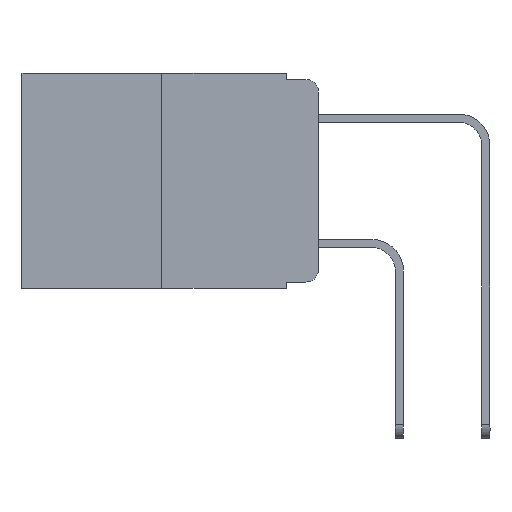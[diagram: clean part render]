
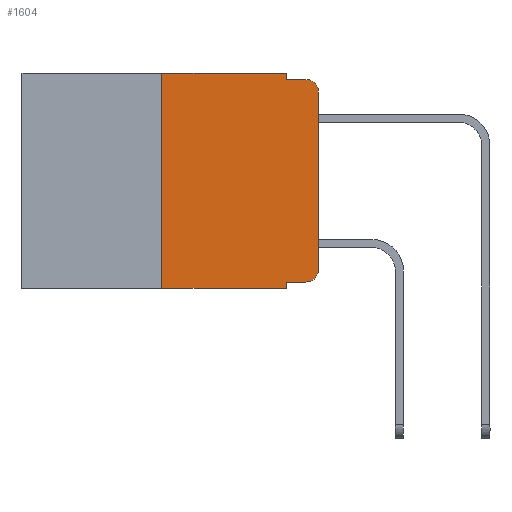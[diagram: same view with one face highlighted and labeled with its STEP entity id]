
A CAD part, left-side view. The second image highlights one B-rep face of the part: STEP entity #1604.
In plain terms, the highlighted planar face has unit normal (-1, 0, 0).
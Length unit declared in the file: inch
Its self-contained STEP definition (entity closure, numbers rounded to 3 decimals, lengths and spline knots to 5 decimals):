
#53 = CARTESIAN_POINT ( 'NONE',  ( 0., 0.473, 0. ) ) ;
#68 = CARTESIAN_POINT ( 'NONE',  ( 0., 0.051, -0.333 ) ) ;
#300 = LINE ( 'NONE', #53, #7227 ) ;
#390 = VERTEX_POINT ( 'NONE', #68 ) ;
#585 = VERTEX_POINT ( 'NONE', #2399 ) ;
#731 = CARTESIAN_POINT ( 'NONE',  ( 0., 0.051, -0.333 ) ) ;
#820 = CARTESIAN_POINT ( 'NONE',  ( 0., 0.051, -0.01 ) ) ;
#1029 = ORIENTED_EDGE ( 'NONE', *, *, #11735, .T. ) ;
#1056 = EDGE_CURVE ( 'NONE', #10828, #585, #1679, .T. ) ;
#1118 = LINE ( 'NONE', #8598, #5354 ) ;
#1265 = CARTESIAN_POINT ( 'NONE',  ( 0., 0.25, -0.343 ) ) ;
#1445 = DIRECTION ( 'NONE',  ( 0., 0., -1. ) ) ;
#1529 = VERTEX_POINT ( 'NONE', #820 ) ;
#1594 = CARTESIAN_POINT ( 'NONE',  ( 0., 0.25, 0. ) ) ;
#1604 = ADVANCED_FACE ( 'NONE', ( #11091 ), #10401, .F. ) ;
#1679 = CIRCLE ( 'NONE', #5750, 0.02 ) ;
#1707 = VECTOR ( 'NONE', #4101, 39.37008 ) ;
#1825 = DIRECTION ( 'NONE',  ( 0., -1., 0. ) ) ;
#1918 = DIRECTION ( 'NONE',  ( 0., 0., -1. ) ) ;
#2091 = CARTESIAN_POINT ( 'NONE',  ( 0., 0.051, -0.343 ) ) ;
#2121 = ORIENTED_EDGE ( 'NONE', *, *, #6467, .T. ) ;
#2207 = CARTESIAN_POINT ( 'NONE',  ( 0., 0.02, -0.333 ) ) ;
#2238 = VECTOR ( 'NONE', #10282, 39.37008 ) ;
#2379 = CARTESIAN_POINT ( 'NONE',  ( 0., 0.25, 0. ) ) ;
#2399 = CARTESIAN_POINT ( 'NONE',  ( 0., 0.02, -0.01 ) ) ;
#2510 = ORIENTED_EDGE ( 'NONE', *, *, #9280, .T. ) ;
#2653 = VECTOR ( 'NONE', #3767, 39.37008 ) ;
#2763 = LINE ( 'NONE', #731, #10683 ) ;
#2851 = ORIENTED_EDGE ( 'NONE', *, *, #8457, .T. ) ;
#3028 = EDGE_CURVE ( 'NONE', #1529, #585, #5027, .T. ) ;
#3047 = VECTOR ( 'NONE', #5261, 39.37008 ) ;
#3082 = EDGE_CURVE ( 'NONE', #390, #3470, #9771, .T. ) ;
#3470 = VERTEX_POINT ( 'NONE', #2091 ) ;
#3767 = DIRECTION ( 'NONE',  ( 0., 0., 1. ) ) ;
#3823 = AXIS2_PLACEMENT_3D ( 'NONE', #9458, #9399, #6631 ) ;
#3838 = DIRECTION ( 'NONE',  ( 0., -1., 0. ) ) ;
#3891 = ORIENTED_EDGE ( 'NONE', *, *, #1056, .T. ) ;
#4101 = DIRECTION ( 'NONE',  ( 0., -1., 0. ) ) ;
#4241 = CARTESIAN_POINT ( 'NONE',  ( 0., 0.051, 0. ) ) ;
#4589 = LINE ( 'NONE', #1594, #3047 ) ;
#4669 = ORIENTED_EDGE ( 'NONE', *, *, #11499, .F. ) ;
#4816 = CARTESIAN_POINT ( 'NONE',  ( 0., 0., 0. ) ) ;
#5027 = LINE ( 'NONE', #7859, #1707 ) ;
#5240 = EDGE_CURVE ( 'NONE', #9430, #7222, #300, .T. ) ;
#5261 = DIRECTION ( 'NONE',  ( 0., 0., 1. ) ) ;
#5354 = VECTOR ( 'NONE', #5616, 39.37008 ) ;
#5549 = CIRCLE ( 'NONE', #3823, 0.02 ) ;
#5616 = DIRECTION ( 'NONE',  ( 0., 0., -1. ) ) ;
#5750 = AXIS2_PLACEMENT_3D ( 'NONE', #10499, #7893, #1445 ) ;
#6467 = EDGE_CURVE ( 'NONE', #390, #8900, #2763, .T. ) ;
#6533 = ORIENTED_EDGE ( 'NONE', *, *, #5240, .F. ) ;
#6602 = CARTESIAN_POINT ( 'NONE',  ( 0., 0.473, -0.343 ) ) ;
#6631 = DIRECTION ( 'NONE',  ( 0., 0., -1. ) ) ;
#6893 = DIRECTION ( 'NONE',  ( 0., 0., -1. ) ) ;
#7222 = VERTEX_POINT ( 'NONE', #4241 ) ;
#7227 = VECTOR ( 'NONE', #3838, 39.37008 ) ;
#7517 = DIRECTION ( 'NONE',  ( 1., 0., 0. ) ) ;
#7696 = CARTESIAN_POINT ( 'NONE',  ( 0., 0.051, 0. ) ) ;
#7859 = CARTESIAN_POINT ( 'NONE',  ( 0., 0.051, -0.01 ) ) ;
#7893 = DIRECTION ( 'NONE',  ( -1., 0., 0. ) ) ;
#7961 = ORIENTED_EDGE ( 'NONE', *, *, #11314, .F. ) ;
#8457 = EDGE_CURVE ( 'NONE', #9432, #3470, #10408, .T. ) ;
#8521 = VECTOR ( 'NONE', #6893, 39.37008 ) ;
#8541 = CARTESIAN_POINT ( 'NONE',  ( 0., 0., -0.313 ) ) ;
#8598 = CARTESIAN_POINT ( 'NONE',  ( 0., 0.051, 0. ) ) ;
#8900 = VERTEX_POINT ( 'NONE', #2207 ) ;
#9247 = CARTESIAN_POINT ( 'NONE',  ( 0., 0.473, 0. ) ) ;
#9259 = ORIENTED_EDGE ( 'NONE', *, *, #3082, .F. ) ;
#9280 = EDGE_CURVE ( 'NONE', #11474, #10828, #9556, .T. ) ;
#9307 = ORIENTED_EDGE ( 'NONE', *, *, #3028, .F. ) ;
#9399 = DIRECTION ( 'NONE',  ( -1., 0., 0. ) ) ;
#9430 = VERTEX_POINT ( 'NONE', #2379 ) ;
#9432 = VERTEX_POINT ( 'NONE', #1265 ) ;
#9458 = CARTESIAN_POINT ( 'NONE',  ( 0., 0.02, -0.313 ) ) ;
#9556 = LINE ( 'NONE', #4816, #2653 ) ;
#9771 = LINE ( 'NONE', #7696, #8521 ) ;
#9902 = EDGE_LOOP ( 'NONE', ( #2510, #3891, #9307, #4669, #6533, #7961, #2851, #9259, #2121, #1029 ) ) ;
#10282 = DIRECTION ( 'NONE',  ( 0., -1., 0. ) ) ;
#10401 = PLANE ( 'NONE',  #11632 ) ;
#10408 = LINE ( 'NONE', #6602, #2238 ) ;
#10499 = CARTESIAN_POINT ( 'NONE',  ( 0., 0.02, -0.03 ) ) ;
#10683 = VECTOR ( 'NONE', #1825, 39.37008 ) ;
#10828 = VERTEX_POINT ( 'NONE', #11038 ) ;
#11038 = CARTESIAN_POINT ( 'NONE',  ( 0., 0., -0.03 ) ) ;
#11091 = FACE_OUTER_BOUND ( 'NONE', #9902, .T. ) ;
#11314 = EDGE_CURVE ( 'NONE', #9432, #9430, #4589, .T. ) ;
#11474 = VERTEX_POINT ( 'NONE', #8541 ) ;
#11499 = EDGE_CURVE ( 'NONE', #7222, #1529, #1118, .T. ) ;
#11632 = AXIS2_PLACEMENT_3D ( 'NONE', #9247, #7517, #1918 ) ;
#11735 = EDGE_CURVE ( 'NONE', #8900, #11474, #5549, .T. ) ;
